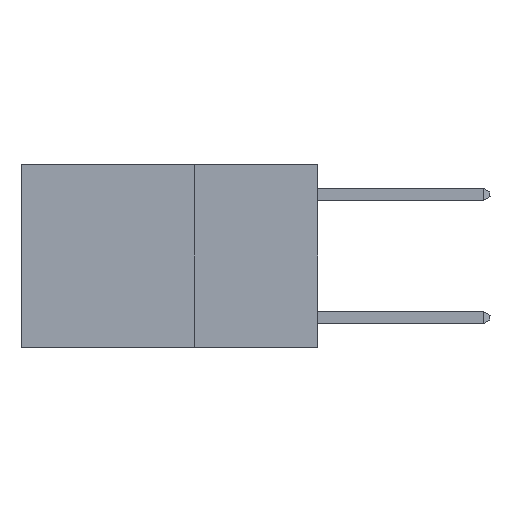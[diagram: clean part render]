
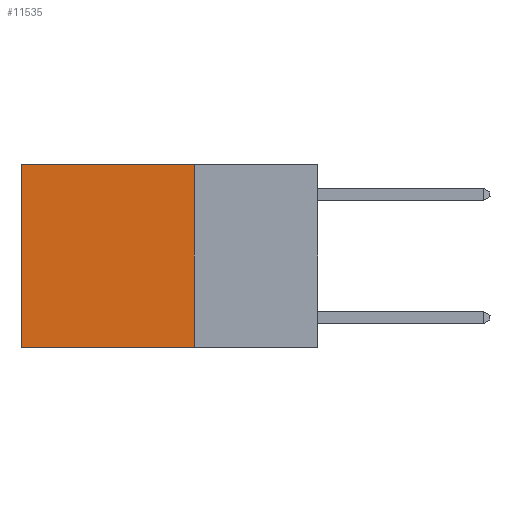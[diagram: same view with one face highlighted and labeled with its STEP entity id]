
A CAD part, left-side view. The second image highlights one B-rep face of the part: STEP entity #11535.
In plain terms, the highlighted planar face has unit normal (-1, 0, 0).
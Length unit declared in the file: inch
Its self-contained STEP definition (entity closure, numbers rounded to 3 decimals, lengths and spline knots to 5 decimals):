
#299 = DIRECTION ( 'NONE',  ( 0., 1., 0. ) ) ;
#1623 = VECTOR ( 'NONE', #26174, 39.37008 ) ;
#3369 = CARTESIAN_POINT ( 'NONE',  ( 0.2625, 0.25, 0. ) ) ;
#4019 = CARTESIAN_POINT ( 'NONE',  ( 0.2625, 0.25, -0.37 ) ) ;
#4499 = EDGE_LOOP ( 'NONE', ( #22241, #8240, #11300, #12252 ) ) ;
#4632 = DIRECTION ( 'NONE',  ( 0., 0., -1. ) ) ;
#5648 = VERTEX_POINT ( 'NONE', #4019 ) ;
#6156 = VERTEX_POINT ( 'NONE', #22736 ) ;
#7076 = DIRECTION ( 'NONE',  ( 0., 1., 0. ) ) ;
#8240 = ORIENTED_EDGE ( 'NONE', *, *, #11802, .F. ) ;
#8521 = CARTESIAN_POINT ( 'NONE',  ( 0.2625, 0.25, 0. ) ) ;
#8857 = EDGE_CURVE ( 'NONE', #12502, #13014, #18201, .T. ) ;
#9391 = FACE_OUTER_BOUND ( 'NONE', #4499, .T. ) ;
#11300 = ORIENTED_EDGE ( 'NONE', *, *, #27077, .F. ) ;
#11535 = ADVANCED_FACE ( 'NONE', ( #9391 ), #21123, .F. ) ;
#11802 = EDGE_CURVE ( 'NONE', #5648, #13014, #14067, .T. ) ;
#12252 = ORIENTED_EDGE ( 'NONE', *, *, #19121, .T. ) ;
#12502 = VERTEX_POINT ( 'NONE', #28577 ) ;
#13014 = VERTEX_POINT ( 'NONE', #25004 ) ;
#14067 = LINE ( 'NONE', #23846, #21007 ) ;
#14103 = CARTESIAN_POINT ( 'NONE',  ( 0.2625, 0.25, 0. ) ) ;
#15899 = DIRECTION ( 'NONE',  ( 0., 0., -1. ) ) ;
#18201 = LINE ( 'NONE', #27556, #21602 ) ;
#19121 = EDGE_CURVE ( 'NONE', #6156, #12502, #28036, .T. ) ;
#21007 = VECTOR ( 'NONE', #299, 39.37008 ) ;
#21123 = PLANE ( 'NONE',  #21954 ) ;
#21602 = VECTOR ( 'NONE', #15899, 39.37008 ) ;
#21868 = LINE ( 'NONE', #3369, #1623 ) ;
#21954 = AXIS2_PLACEMENT_3D ( 'NONE', #8521, #25717, #4632 ) ;
#22241 = ORIENTED_EDGE ( 'NONE', *, *, #8857, .T. ) ;
#22736 = CARTESIAN_POINT ( 'NONE',  ( 0.2625, 0.25, 0. ) ) ;
#23846 = CARTESIAN_POINT ( 'NONE',  ( 0.2625, 0.25, -0.37 ) ) ;
#25004 = CARTESIAN_POINT ( 'NONE',  ( 0.2625, 0.6, -0.37 ) ) ;
#25717 = DIRECTION ( 'NONE',  ( 1., 0., 0. ) ) ;
#26174 = DIRECTION ( 'NONE',  ( 0., 0., -1. ) ) ;
#27077 = EDGE_CURVE ( 'NONE', #6156, #5648, #21868, .T. ) ;
#27556 = CARTESIAN_POINT ( 'NONE',  ( 0.2625, 0.6, 0. ) ) ;
#27726 = VECTOR ( 'NONE', #7076, 39.37008 ) ;
#28036 = LINE ( 'NONE', #14103, #27726 ) ;
#28577 = CARTESIAN_POINT ( 'NONE',  ( 0.2625, 0.6, 0. ) ) ;
